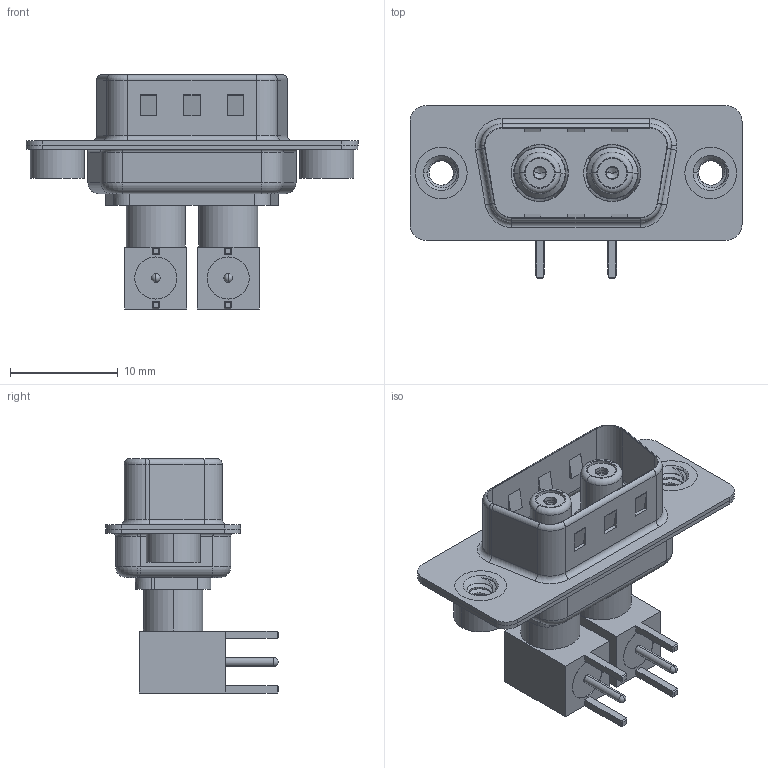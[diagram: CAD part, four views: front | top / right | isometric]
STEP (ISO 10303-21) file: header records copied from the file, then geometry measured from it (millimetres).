
FILE_DESCRIPTION (( 'STEP AP203' ), '1' );
FILE_NAME ('629-2W2-640-7N2.STEP', '2022-05-04T22:52:50', ( '' ), ( '' ), 'SwSTEP 2.0', 'SolidWorks 2020', '' );
FILE_SCHEMA (( 'CONFIG_CONTROL_DESIGN' ));
Length unit declared in the file: millimetre
Products named in the file (14): Socket_RA; 629Combo Housing_2W2; Co-Ax Jack Assy_RA; Insulator RA Pin; 629Combo Threaded Rivet_2; 629Combo Shell Rear_09 Contacts; 629-2W2-640-7N2; RA Back Shell; 629Combo Shell Front_09 Contacts; Locking Collar; Insulator Socket; Co-Ax Jack_RA PC Tail; Insulator Socket 2
Assembly tree (21 placements, depth 3):
  629-2W2-640-7N2
    629Combo Housing_2W2
    629Combo Shell Rear_09 Contacts
    629Combo Shell Front_09 Contacts
    629Combo Threaded Rivet_2  x2
    Co-Ax Jack Assy_RA
      Co-Ax Jack_RA PC Tail
      Insulator Socket
      Insulator Socket 2
      Locking Collar
      Socket_RA
      RA Back Shell
      Insulator RA Pin
    Co-Ax Jack Assy_RA
      Co-Ax Jack_RA PC Tail
      Insulator Socket
      Insulator Socket 2
      Locking Collar
      Socket_RA
      RA Back Shell
      Insulator RA Pin
Bounding box: 30.8 x 16 x 21.71 mm (x, y, z)
Volume: 1883.5 mm3; surface area: 5464.5 mm2
Topology: 19 solids, 19 shells, 608 faces, 1447 edges, 900 vertices
Faces by surface type: cylinder 263, plane 221, torus 62, cone 50, bspline 8, sphere 4
Entity records: 15807 total; most frequent: CARTESIAN_POINT 3846, DIRECTION 2298, ORIENTED_EDGE 2042, EDGE_CURVE 1021, AXIS2_PLACEMENT_3D 892, VERTEX_POINT 641, VECTOR 514, LINE 514
